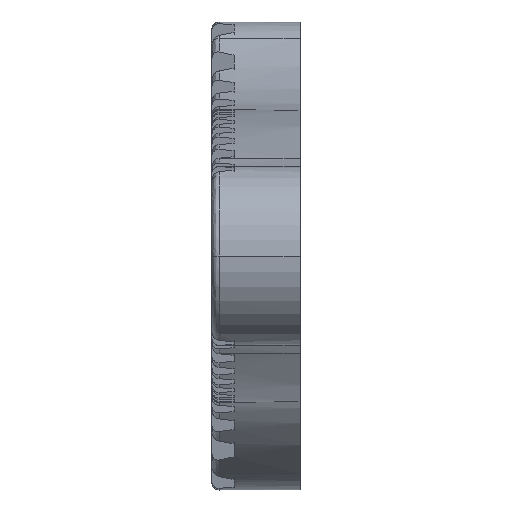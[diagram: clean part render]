
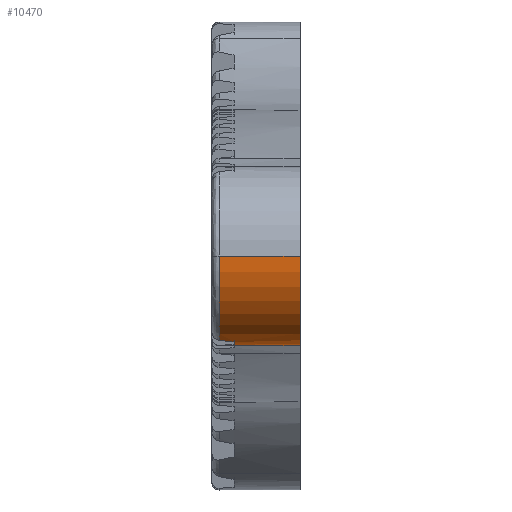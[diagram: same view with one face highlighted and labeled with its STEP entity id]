
A CAD part, front view. The second image highlights one B-rep face of the part: STEP entity #10470.
In plain terms, the highlighted cylindrical face has radius 12.15 mm (diameter 24.3 mm), a partial arc.
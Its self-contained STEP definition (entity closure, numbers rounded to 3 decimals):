
#2 = AXIS2_PLACEMENT_3D ( 'NONE', #8528, #8467, #12402 ) ;
#78 = VERTEX_POINT ( 'NONE', #3445 ) ;
#352 = EDGE_CURVE ( 'NONE', #10806, #9072, #4206, .T. ) ;
#640 = VERTEX_POINT ( 'NONE', #8425 ) ;
#1173 = ORIENTED_EDGE ( 'NONE', *, *, #12319, .T. ) ;
#1181 = CARTESIAN_POINT ( 'NONE',  ( -440.582, -90.237, -10.582 ) ) ;
#1344 = CARTESIAN_POINT ( 'NONE',  ( -431.682, -86.722, 1.048 ) ) ;
#1400 = CARTESIAN_POINT ( 'NONE',  ( -442.364, -84.885, -10.962 ) ) ;
#1841 = CARTESIAN_POINT ( 'NONE',  ( -442.582, -90.903, -10.36 ) ) ;
#2026 = CARTESIAN_POINT ( 'NONE',  ( -441.922, -90.683, -10.44 ) ) ;
#2106 = CARTESIAN_POINT ( 'NONE',  ( -404.682, -98.872, 1. ) ) ;
#2115 = DIRECTION ( 'NONE',  ( 0., -1., 0. ) ) ;
#2165 = DIRECTION ( 'NONE',  ( 0., -1., 0. ) ) ;
#2276 = CARTESIAN_POINT ( 'NONE',  ( -441.246, -88.597, -10.958 ) ) ;
#2366 = CARTESIAN_POINT ( 'NONE',  ( -442.582, -84.958, -10.973 ) ) ;
#2642 = VERTEX_POINT ( 'NONE', #9566 ) ;
#2781 = EDGE_CURVE ( 'NONE', #640, #10012, #7805, .T. ) ;
#2817 = LINE ( 'NONE', #2106, #5999 ) ;
#2827 = FACE_OUTER_BOUND ( 'NONE', #5560, .T. ) ;
#3006 = EDGE_CURVE ( 'NONE', #640, #5082, #12330, .T. ) ;
#3250 = ORIENTED_EDGE ( 'NONE', *, *, #4607, .T. ) ;
#3253 = DIRECTION ( 'NONE',  ( 0., -1., 0. ) ) ;
#3278 = ORIENTED_EDGE ( 'NONE', *, *, #3404, .T. ) ;
#3404 = EDGE_CURVE ( 'NONE', #2642, #10806, #3808, .T. ) ;
#3445 = CARTESIAN_POINT ( 'NONE',  ( -440.582, -88.818, -10.92 ) ) ;
#3808 = CIRCLE ( 'NONE', #6447, 12.15 ) ;
#3981 = ORIENTED_EDGE ( 'NONE', *, *, #3006, .F. ) ;
#4206 =( BOUNDED_CURVE ( )  B_SPLINE_CURVE ( 3, ( #10725, #2026, #9891, #1181 ),
 .UNSPECIFIED., .F., .T. ) 
 B_SPLINE_CURVE_WITH_KNOTS ( ( 4, 4 ),
 ( 1.219, 1.277 ),
 .UNSPECIFIED. ) 
 CURVE ( )  GEOMETRIC_REPRESENTATION_ITEM ( )  RATIONAL_B_SPLINE_CURVE ( ( 1., 1., 1., 1. ) ) 
 REPRESENTATION_ITEM ( '' )  );
#4211 = DIRECTION ( 'NONE',  ( 1., 0., 0. ) ) ;
#4567 = AXIS2_PLACEMENT_3D ( 'NONE', #1344, #7080, #11960 ) ;
#4607 = EDGE_CURVE ( 'NONE', #78, #6406, #7066, .T. ) ;
#4795 = CARTESIAN_POINT ( 'NONE',  ( -431.682, -98.872, 1. ) ) ;
#5082 = VERTEX_POINT ( 'NONE', #10250 ) ;
#5174 = CARTESIAN_POINT ( 'NONE',  ( -404.682, -86.722, 1.048 ) ) ;
#5524 = CIRCLE ( 'NONE', #2, 12.15 ) ;
#5560 = EDGE_LOOP ( 'NONE', ( #1173, #3250, #6865, #3981, #7940, #5970, #9186, #3278, #10859 ) ) ;
#5565 = CIRCLE ( 'NONE', #4567, 12.15 ) ;
#5970 = ORIENTED_EDGE ( 'NONE', *, *, #7369, .F. ) ;
#5999 = VECTOR ( 'NONE', #10744, 1000. ) ;
#6143 = CARTESIAN_POINT ( 'NONE',  ( -440.582, -88.818, -10.92 ) ) ;
#6406 = VERTEX_POINT ( 'NONE', #8354 ) ;
#6447 = AXIS2_PLACEMENT_3D ( 'NONE', #12580, #4211, #3253 ) ;
#6646 = DIRECTION ( 'NONE',  ( -1., 0., 0. ) ) ;
#6656 = VECTOR ( 'NONE', #7035, 1000. ) ;
#6865 = ORIENTED_EDGE ( 'NONE', *, *, #9220, .T. ) ;
#7035 = DIRECTION ( 'NONE',  ( 1., 0., 0. ) ) ;
#7066 =( BOUNDED_CURVE ( )  B_SPLINE_CURVE ( 3, ( #6143, #2276, #8879, #10018 ),
 .UNSPECIFIED., .F., .T. ) 
 B_SPLINE_CURVE_WITH_KNOTS ( ( 4, 4 ),
 ( 4.539, 4.595 ),
 .UNSPECIFIED. ) 
 CURVE ( )  GEOMETRIC_REPRESENTATION_ITEM ( )  RATIONAL_B_SPLINE_CURVE ( ( 1., 1., 1., 1. ) ) 
 REPRESENTATION_ITEM ( '' )  );
#7080 = DIRECTION ( 'NONE',  ( 1., 0., 0. ) ) ;
#7369 = EDGE_CURVE ( 'NONE', #11489, #10012, #5565, .T. ) ;
#7705 = EDGE_CURVE ( 'NONE', #11489, #2642, #2817, .T. ) ;
#7805 = LINE ( 'NONE', #9757, #6656 ) ;
#7940 = ORIENTED_EDGE ( 'NONE', *, *, #2781, .T. ) ;
#8056 = CARTESIAN_POINT ( 'NONE',  ( -431.682, -84.74, -10.939 ) ) ;
#8354 = CARTESIAN_POINT ( 'NONE',  ( -442.582, -88.151, -11.017 ) ) ;
#8425 = CARTESIAN_POINT ( 'NONE',  ( -441.929, -84.74, -10.939 ) ) ;
#8467 = DIRECTION ( 'NONE',  ( 1., 0., 0. ) ) ;
#8528 = CARTESIAN_POINT ( 'NONE',  ( -440.582, -86.722, 1.048 ) ) ;
#8599 = CARTESIAN_POINT ( 'NONE',  ( -440.582, -90.237, -10.582 ) ) ;
#8789 = DIRECTION ( 'NONE',  ( 1., 0., 0. ) ) ;
#8879 = CARTESIAN_POINT ( 'NONE',  ( -441.913, -88.374, -10.991 ) ) ;
#8957 = CYLINDRICAL_SURFACE ( 'NONE', #11354, 12.15 ) ;
#9064 = CIRCLE ( 'NONE', #11902, 12.15 ) ;
#9072 = VERTEX_POINT ( 'NONE', #8599 ) ;
#9186 = ORIENTED_EDGE ( 'NONE', *, *, #7705, .T. ) ;
#9220 = EDGE_CURVE ( 'NONE', #6406, #5082, #9064, .T. ) ;
#9566 = CARTESIAN_POINT ( 'NONE',  ( -442.582, -98.872, 1. ) ) ;
#9757 = CARTESIAN_POINT ( 'NONE',  ( -404.682, -84.74, -10.939 ) ) ;
#9891 = CARTESIAN_POINT ( 'NONE',  ( -441.255, -90.461, -10.514 ) ) ;
#10012 = VERTEX_POINT ( 'NONE', #8056 ) ;
#10018 = CARTESIAN_POINT ( 'NONE',  ( -442.582, -88.151, -11.017 ) ) ;
#10250 = CARTESIAN_POINT ( 'NONE',  ( -442.582, -84.958, -10.973 ) ) ;
#10470 = ADVANCED_FACE ( 'NONE', ( #2827 ), #8957, .T. ) ;
#10725 = CARTESIAN_POINT ( 'NONE',  ( -442.582, -90.903, -10.36 ) ) ;
#10744 = DIRECTION ( 'NONE',  ( -1., 0., 0. ) ) ;
#10806 = VERTEX_POINT ( 'NONE', #1841 ) ;
#10812 = CARTESIAN_POINT ( 'NONE',  ( -442.146, -84.812, -10.951 ) ) ;
#10816 = CARTESIAN_POINT ( 'NONE',  ( -442.582, -86.722, 1.048 ) ) ;
#10859 = ORIENTED_EDGE ( 'NONE', *, *, #352, .T. ) ;
#11354 = AXIS2_PLACEMENT_3D ( 'NONE', #5174, #6646, #2165 ) ;
#11489 = VERTEX_POINT ( 'NONE', #4795 ) ;
#11887 = CARTESIAN_POINT ( 'NONE',  ( -441.929, -84.74, -10.939 ) ) ;
#11902 = AXIS2_PLACEMENT_3D ( 'NONE', #10816, #8789, #2115 ) ;
#11960 = DIRECTION ( 'NONE',  ( 0., 1., 0. ) ) ;
#12319 = EDGE_CURVE ( 'NONE', #9072, #78, #5524, .T. ) ;
#12330 =( BOUNDED_CURVE ( )  B_SPLINE_CURVE ( 3, ( #11887, #10812, #1400, #2366 ),
 .UNSPECIFIED., .F., .T. ) 
 B_SPLINE_CURVE_WITH_KNOTS ( ( 4, 4 ),
 ( 4.548, 4.567 ),
 .UNSPECIFIED. ) 
 CURVE ( )  GEOMETRIC_REPRESENTATION_ITEM ( )  RATIONAL_B_SPLINE_CURVE ( ( 1., 1., 1., 1. ) ) 
 REPRESENTATION_ITEM ( '' )  );
#12402 = DIRECTION ( 'NONE',  ( 0., -1., 0. ) ) ;
#12580 = CARTESIAN_POINT ( 'NONE',  ( -442.582, -86.722, 1.048 ) ) ;
